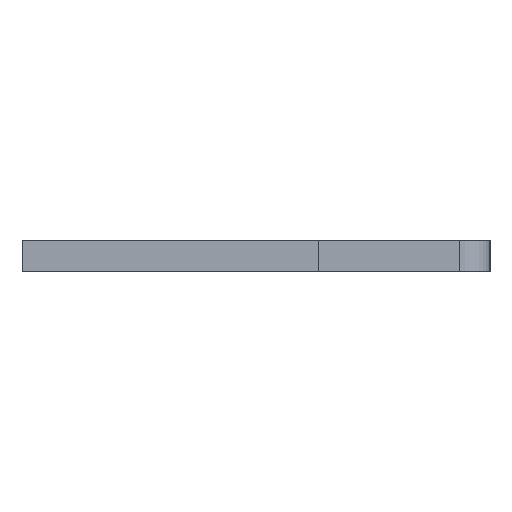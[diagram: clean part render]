
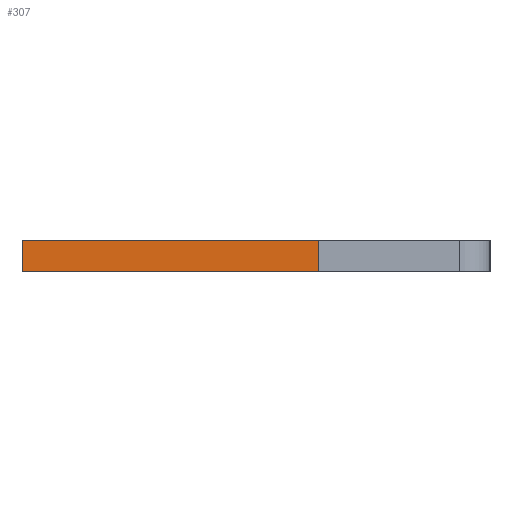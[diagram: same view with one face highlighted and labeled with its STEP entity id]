
A CAD part, left-side view. The second image highlights one B-rep face of the part: STEP entity #307.
In plain terms, the highlighted face is planar.
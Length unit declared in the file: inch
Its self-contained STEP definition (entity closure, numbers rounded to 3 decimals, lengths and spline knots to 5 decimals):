
#112 = LINE ( 'NONE', #1689, #1098 ) ;
#123 = LINE ( 'NONE', #1805, #1822 ) ;
#270 = CARTESIAN_POINT ( 'NONE',  ( 0.01, 0.15, -0.04 ) ) ;
#307 = ADVANCED_FACE ( 'NONE', ( #1967 ), #664, .F. ) ;
#404 = DIRECTION ( 'NONE',  ( -1., 0., 0. ) ) ;
#546 = LINE ( 'NONE', #1942, #1717 ) ;
#552 = VERTEX_POINT ( 'NONE', #1568 ) ;
#565 = DIRECTION ( 'NONE',  ( -1., 0., 0. ) ) ;
#664 = PLANE ( 'NONE',  #988 ) ;
#681 = ORIENTED_EDGE ( 'NONE', *, *, #1154, .F. ) ;
#752 = DIRECTION ( 'NONE',  ( 0., 1., 0. ) ) ;
#815 = DIRECTION ( 'NONE',  ( 0., 0., 1. ) ) ;
#988 = AXIS2_PLACEMENT_3D ( 'NONE', #1736, #815, #1874 ) ;
#1018 = EDGE_CURVE ( 'NONE', #552, #1378, #123, .T. ) ;
#1024 = CARTESIAN_POINT ( 'NONE',  ( 0.01, 0.15, -0.04 ) ) ;
#1096 = VERTEX_POINT ( 'NONE', #1024 ) ;
#1098 = VECTOR ( 'NONE', #1407, 39.37008 ) ;
#1154 = EDGE_CURVE ( 'NONE', #1096, #1192, #546, .T. ) ;
#1192 = VERTEX_POINT ( 'NONE', #1774 ) ;
#1202 = VECTOR ( 'NONE', #752, 39.37008 ) ;
#1300 = ORIENTED_EDGE ( 'NONE', *, *, #1928, .T. ) ;
#1325 = ORIENTED_EDGE ( 'NONE', *, *, #1018, .T. ) ;
#1336 = CARTESIAN_POINT ( 'NONE',  ( -0.01, -0.04, -0.04 ) ) ;
#1378 = VERTEX_POINT ( 'NONE', #1336 ) ;
#1407 = DIRECTION ( 'NONE',  ( 0., 1., 0. ) ) ;
#1568 = CARTESIAN_POINT ( 'NONE',  ( 0.01, -0.04, -0.04 ) ) ;
#1689 = CARTESIAN_POINT ( 'NONE',  ( -0.01, 0.15, -0.04 ) ) ;
#1717 = VECTOR ( 'NONE', #565, 39.37008 ) ;
#1720 = LINE ( 'NONE', #270, #1202 ) ;
#1736 = CARTESIAN_POINT ( 'NONE',  ( 0.01, 0.15, -0.04 ) ) ;
#1756 = EDGE_CURVE ( 'NONE', #552, #1096, #1720, .T. ) ;
#1774 = CARTESIAN_POINT ( 'NONE',  ( -0.01, 0.15, -0.04 ) ) ;
#1805 = CARTESIAN_POINT ( 'NONE',  ( 0.01, -0.04, -0.04 ) ) ;
#1822 = VECTOR ( 'NONE', #404, 39.37008 ) ;
#1833 = ORIENTED_EDGE ( 'NONE', *, *, #1756, .F. ) ;
#1834 = EDGE_LOOP ( 'NONE', ( #1300, #681, #1833, #1325 ) ) ;
#1874 = DIRECTION ( 'NONE',  ( 1., 0., 0. ) ) ;
#1928 = EDGE_CURVE ( 'NONE', #1378, #1192, #112, .T. ) ;
#1942 = CARTESIAN_POINT ( 'NONE',  ( 0.01, 0.15, -0.04 ) ) ;
#1967 = FACE_OUTER_BOUND ( 'NONE', #1834, .T. ) ;
